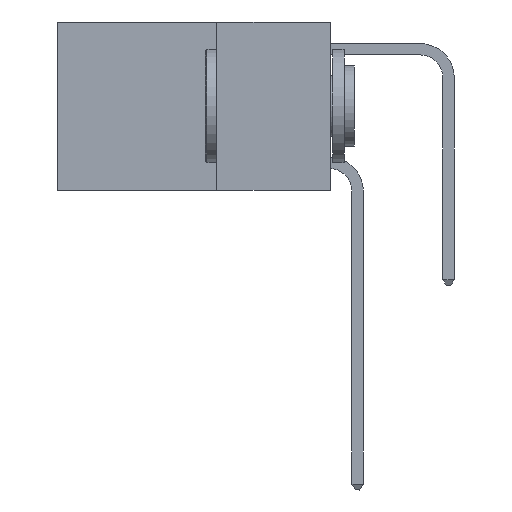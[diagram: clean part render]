
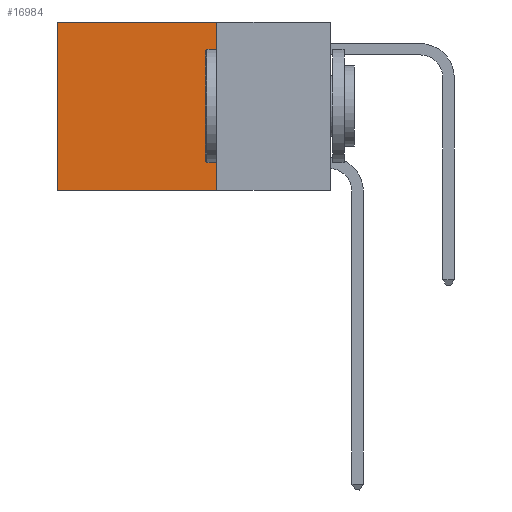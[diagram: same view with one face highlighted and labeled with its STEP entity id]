
A CAD part, left-side view. The second image highlights one B-rep face of the part: STEP entity #16984.
In plain terms, the highlighted planar face has unit normal (-1, 0, 0).
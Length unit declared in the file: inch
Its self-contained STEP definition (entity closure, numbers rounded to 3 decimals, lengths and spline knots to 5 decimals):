
#111 = DIRECTION ( 'NONE',  ( 0., 1., 0. ) ) ;
#256 = CARTESIAN_POINT ( 'NONE',  ( 0.2625, 0.6, -0.37 ) ) ;
#1181 = EDGE_LOOP ( 'NONE', ( #21170, #22133, #20637, #7006 ) ) ;
#1313 = VERTEX_POINT ( 'NONE', #256 ) ;
#1592 = CARTESIAN_POINT ( 'NONE',  ( 0.2625, 0.25, -0.37 ) ) ;
#2109 = CARTESIAN_POINT ( 'NONE',  ( 0.2625, 0.25, 0. ) ) ;
#4060 = EDGE_CURVE ( 'NONE', #25087, #5121, #25470, .T. ) ;
#4350 = LINE ( 'NONE', #17581, #25372 ) ;
#5121 = VERTEX_POINT ( 'NONE', #24678 ) ;
#7006 = ORIENTED_EDGE ( 'NONE', *, *, #4060, .T. ) ;
#7235 = CARTESIAN_POINT ( 'NONE',  ( 0.2625, 0.6, 0. ) ) ;
#8029 = DIRECTION ( 'NONE',  ( 0., 1., 0. ) ) ;
#8773 = VECTOR ( 'NONE', #111, 39.37008 ) ;
#9399 = DIRECTION ( 'NONE',  ( 0., 0., -1. ) ) ;
#10024 = VERTEX_POINT ( 'NONE', #12082 ) ;
#10671 = DIRECTION ( 'NONE',  ( 0., 0., -1. ) ) ;
#11351 = DIRECTION ( 'NONE',  ( 0., 0., -1. ) ) ;
#12082 = CARTESIAN_POINT ( 'NONE',  ( 0.2625, 0.25, -0.37 ) ) ;
#12526 = EDGE_CURVE ( 'NONE', #10024, #1313, #13526, .T. ) ;
#12881 = VECTOR ( 'NONE', #8029, 39.37008 ) ;
#13526 = LINE ( 'NONE', #1592, #12881 ) ;
#13836 = AXIS2_PLACEMENT_3D ( 'NONE', #2109, #23186, #10671 ) ;
#16567 = EDGE_CURVE ( 'NONE', #5121, #1313, #26242, .T. ) ;
#16984 = ADVANCED_FACE ( 'NONE', ( #20673 ), #21098, .F. ) ;
#17581 = CARTESIAN_POINT ( 'NONE',  ( 0.2625, 0.25, 0. ) ) ;
#20637 = ORIENTED_EDGE ( 'NONE', *, *, #25571, .F. ) ;
#20673 = FACE_OUTER_BOUND ( 'NONE', #1181, .T. ) ;
#21098 = PLANE ( 'NONE',  #13836 ) ;
#21170 = ORIENTED_EDGE ( 'NONE', *, *, #16567, .T. ) ;
#22133 = ORIENTED_EDGE ( 'NONE', *, *, #12526, .F. ) ;
#23186 = DIRECTION ( 'NONE',  ( 1., 0., 0. ) ) ;
#24143 = CARTESIAN_POINT ( 'NONE',  ( 0.2625, 0.25, 0. ) ) ;
#24678 = CARTESIAN_POINT ( 'NONE',  ( 0.2625, 0.6, 0. ) ) ;
#25087 = VERTEX_POINT ( 'NONE', #24143 ) ;
#25358 = CARTESIAN_POINT ( 'NONE',  ( 0.2625, 0.25, 0. ) ) ;
#25372 = VECTOR ( 'NONE', #11351, 39.37008 ) ;
#25470 = LINE ( 'NONE', #25358, #8773 ) ;
#25571 = EDGE_CURVE ( 'NONE', #25087, #10024, #4350, .T. ) ;
#25585 = VECTOR ( 'NONE', #9399, 39.37008 ) ;
#26242 = LINE ( 'NONE', #7235, #25585 ) ;
